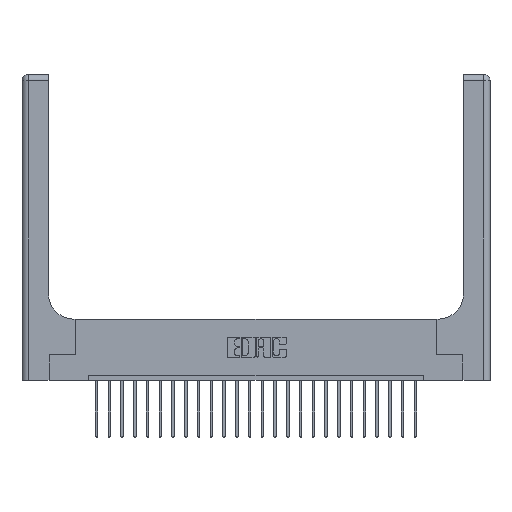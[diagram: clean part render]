
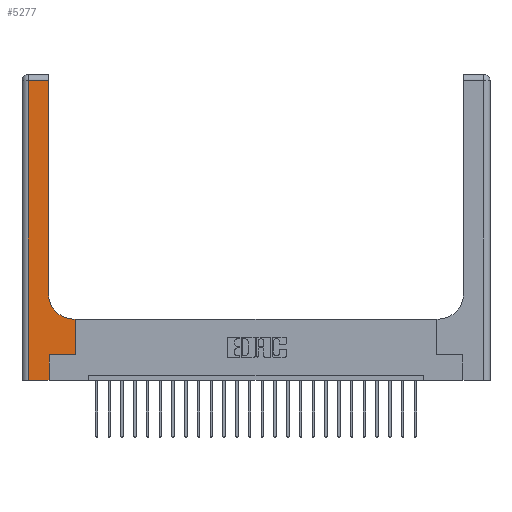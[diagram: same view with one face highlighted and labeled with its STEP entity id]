
A CAD part, top view. The second image highlights one B-rep face of the part: STEP entity #5277.
In plain terms, the highlighted planar face has unit normal (0, 0, 1).
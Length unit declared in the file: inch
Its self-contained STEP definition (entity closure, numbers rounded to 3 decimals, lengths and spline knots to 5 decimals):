
#603 = ORIENTED_EDGE ( 'NONE', *, *, #18702, .T. ) ;
#606 = CARTESIAN_POINT ( 'NONE',  ( 0.26, 0.85, 0.37 ) ) ;
#2478 = EDGE_CURVE ( 'NONE', #16083, #3194, #23601, .T. ) ;
#3032 = LINE ( 'NONE', #11874, #14290 ) ;
#3194 = VERTEX_POINT ( 'NONE', #22810 ) ;
#3246 = EDGE_LOOP ( 'NONE', ( #7089, #7156, #9817, #15763, #14599, #10467, #603, #18063, #23275 ) ) ;
#3558 = EDGE_CURVE ( 'NONE', #17708, #13713, #20622, .T. ) ;
#3861 = LINE ( 'NONE', #9422, #16900 ) ;
#4146 = VECTOR ( 'NONE', #12567, 39.37008 ) ;
#4165 = DIRECTION ( 'NONE',  ( 0., 0., -1. ) ) ;
#4906 = VERTEX_POINT ( 'NONE', #13732 ) ;
#5025 = DIRECTION ( 'NONE',  ( 1., 0., 0. ) ) ;
#5277 = ADVANCED_FACE ( 'NONE', ( #14567 ), #23127, .F. ) ;
#5670 = CARTESIAN_POINT ( 'NONE',  ( 0.265, 0.25, 0.37 ) ) ;
#6245 = CARTESIAN_POINT ( 'NONE',  ( 0.265, 0., 0.37 ) ) ;
#6305 = DIRECTION ( 'NONE',  ( -1., 0., 0. ) ) ;
#6874 = CARTESIAN_POINT ( 'NONE',  ( 0.265, 0.25, 0.37 ) ) ;
#7038 = LINE ( 'NONE', #21935, #11143 ) ;
#7089 = ORIENTED_EDGE ( 'NONE', *, *, #17478, .T. ) ;
#7111 = VERTEX_POINT ( 'NONE', #606 ) ;
#7156 = ORIENTED_EDGE ( 'NONE', *, *, #3558, .T. ) ;
#7426 = CARTESIAN_POINT ( 'NONE',  ( 0.51, 0.85, 0.37 ) ) ;
#7564 = VECTOR ( 'NONE', #11810, 39.37008 ) ;
#7748 = CARTESIAN_POINT ( 'NONE',  ( 0.06, 3., 0.37 ) ) ;
#8351 = CARTESIAN_POINT ( 'NONE',  ( 0., 3., 0.37 ) ) ;
#8418 = LINE ( 'NONE', #16026, #10654 ) ;
#9311 = VECTOR ( 'NONE', #14804, 39.37008 ) ;
#9422 = CARTESIAN_POINT ( 'NONE',  ( 0.26, 3., 0.37 ) ) ;
#9691 = LINE ( 'NONE', #7748, #12595 ) ;
#9817 = ORIENTED_EDGE ( 'NONE', *, *, #15754, .T. ) ;
#10385 = CIRCLE ( 'NONE', #15027, 0.25 ) ;
#10467 = ORIENTED_EDGE ( 'NONE', *, *, #2478, .T. ) ;
#10654 = VECTOR ( 'NONE', #5025, 39.37008 ) ;
#11143 = VECTOR ( 'NONE', #14657, 39.37008 ) ;
#11179 = DIRECTION ( 'NONE',  ( 1., 0., 0. ) ) ;
#11698 = LINE ( 'NONE', #6245, #7564 ) ;
#11810 = DIRECTION ( 'NONE',  ( 0., 1., 0. ) ) ;
#11874 = CARTESIAN_POINT ( 'NONE',  ( 0.26, 0.6, 0.37 ) ) ;
#12252 = AXIS2_PLACEMENT_3D ( 'NONE', #8351, #4165, #13355 ) ;
#12567 = DIRECTION ( 'NONE',  ( 1., 0., 0. ) ) ;
#12595 = VECTOR ( 'NONE', #15132, 39.37008 ) ;
#12677 = CARTESIAN_POINT ( 'NONE',  ( 0.06, 0., 0.37 ) ) ;
#13355 = DIRECTION ( 'NONE',  ( -1., 0., 0. ) ) ;
#13713 = VERTEX_POINT ( 'NONE', #15474 ) ;
#13732 = CARTESIAN_POINT ( 'NONE',  ( 0.51, 0.6, 0.37 ) ) ;
#14169 = EDGE_CURVE ( 'NONE', #20362, #16083, #11698, .T. ) ;
#14246 = EDGE_CURVE ( 'NONE', #21609, #20362, #8418, .T. ) ;
#14290 = VECTOR ( 'NONE', #6305, 39.37008 ) ;
#14567 = FACE_OUTER_BOUND ( 'NONE', #3246, .T. ) ;
#14599 = ORIENTED_EDGE ( 'NONE', *, *, #14169, .T. ) ;
#14657 = DIRECTION ( 'NONE',  ( 0., 1., 0. ) ) ;
#14804 = DIRECTION ( 'NONE',  ( -1., 0., 0. ) ) ;
#14805 = DIRECTION ( 'NONE',  ( 0., 0., -1. ) ) ;
#15027 = AXIS2_PLACEMENT_3D ( 'NONE', #7426, #14805, #11179 ) ;
#15041 = CARTESIAN_POINT ( 'NONE',  ( 0., 2.94, 0.37 ) ) ;
#15132 = DIRECTION ( 'NONE',  ( 0., -1., 0. ) ) ;
#15474 = CARTESIAN_POINT ( 'NONE',  ( 0.06, 2.94, 0.37 ) ) ;
#15754 = EDGE_CURVE ( 'NONE', #13713, #21609, #9691, .T. ) ;
#15763 = ORIENTED_EDGE ( 'NONE', *, *, #14246, .T. ) ;
#16026 = CARTESIAN_POINT ( 'NONE',  ( 0., 0., 0.37 ) ) ;
#16083 = VERTEX_POINT ( 'NONE', #5670 ) ;
#16804 = DIRECTION ( 'NONE',  ( 0., 1., 0. ) ) ;
#16900 = VECTOR ( 'NONE', #16804, 39.37008 ) ;
#17478 = EDGE_CURVE ( 'NONE', #7111, #17708, #3861, .T. ) ;
#17708 = VERTEX_POINT ( 'NONE', #19684 ) ;
#18063 = ORIENTED_EDGE ( 'NONE', *, *, #22339, .T. ) ;
#18702 = EDGE_CURVE ( 'NONE', #3194, #18864, #7038, .T. ) ;
#18864 = VERTEX_POINT ( 'NONE', #22411 ) ;
#19436 = EDGE_CURVE ( 'NONE', #4906, #7111, #10385, .T. ) ;
#19684 = CARTESIAN_POINT ( 'NONE',  ( 0.26, 2.94, 0.37 ) ) ;
#20362 = VERTEX_POINT ( 'NONE', #22621 ) ;
#20622 = LINE ( 'NONE', #15041, #9311 ) ;
#21609 = VERTEX_POINT ( 'NONE', #12677 ) ;
#21935 = CARTESIAN_POINT ( 'NONE',  ( 0.528, 0.25, 0.37 ) ) ;
#22339 = EDGE_CURVE ( 'NONE', #18864, #4906, #3032, .T. ) ;
#22411 = CARTESIAN_POINT ( 'NONE',  ( 0.528, 0.6, 0.37 ) ) ;
#22621 = CARTESIAN_POINT ( 'NONE',  ( 0.265, 0., 0.37 ) ) ;
#22810 = CARTESIAN_POINT ( 'NONE',  ( 0.528, 0.25, 0.37 ) ) ;
#23127 = PLANE ( 'NONE',  #12252 ) ;
#23275 = ORIENTED_EDGE ( 'NONE', *, *, #19436, .T. ) ;
#23601 = LINE ( 'NONE', #6874, #4146 ) ;
